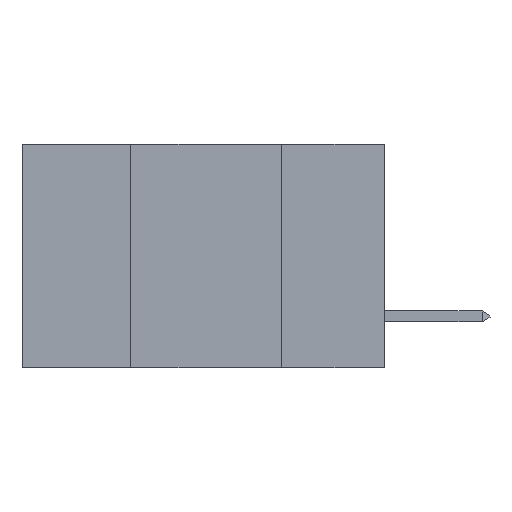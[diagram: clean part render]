
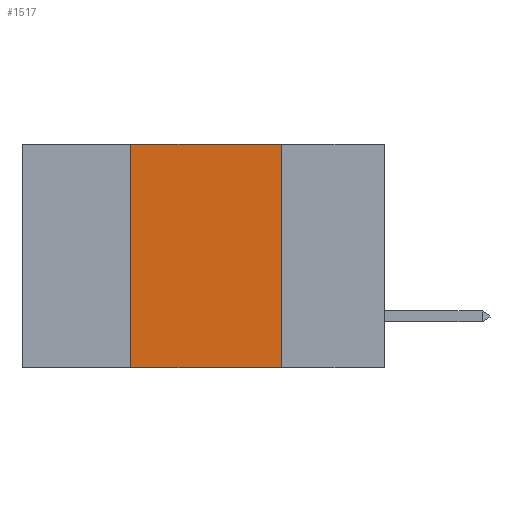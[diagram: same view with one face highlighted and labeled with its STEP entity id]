
A CAD part, left-side view. The second image highlights one B-rep face of the part: STEP entity #1517.
In plain terms, the highlighted planar face has unit normal (-1, 0, 0).
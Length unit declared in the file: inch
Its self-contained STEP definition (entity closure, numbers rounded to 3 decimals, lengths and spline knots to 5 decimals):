
#461 = CARTESIAN_POINT ( 'NONE',  ( 0., 0.6, 0. ) ) ;
#580 = EDGE_CURVE ( 'NONE', #10072, #6697, #18941, .T. ) ;
#1517 = ADVANCED_FACE ( 'NONE', ( #11629 ), #19166, .F. ) ;
#2607 = CARTESIAN_POINT ( 'NONE',  ( 0., 0.42, 0. ) ) ;
#3181 = VECTOR ( 'NONE', #10571, 39.37008 ) ;
#3670 = LINE ( 'NONE', #6433, #8417 ) ;
#4183 = EDGE_CURVE ( 'NONE', #6176, #10072, #11849, .T. ) ;
#5611 = DIRECTION ( 'NONE',  ( 0., -1., 0. ) ) ;
#6176 = VERTEX_POINT ( 'NONE', #2607 ) ;
#6433 = CARTESIAN_POINT ( 'NONE',  ( 0., 0.6, -0.37 ) ) ;
#6697 = VERTEX_POINT ( 'NONE', #12867 ) ;
#7623 = VECTOR ( 'NONE', #19845, 39.37008 ) ;
#8417 = VECTOR ( 'NONE', #20588, 39.37008 ) ;
#8633 = CARTESIAN_POINT ( 'NONE',  ( 0., 0.42, 0. ) ) ;
#8775 = ORIENTED_EDGE ( 'NONE', *, *, #20152, .F. ) ;
#9837 = ORIENTED_EDGE ( 'NONE', *, *, #13839, .T. ) ;
#10072 = VERTEX_POINT ( 'NONE', #19743 ) ;
#10571 = DIRECTION ( 'NONE',  ( 0., 0., -1. ) ) ;
#11629 = FACE_OUTER_BOUND ( 'NONE', #12415, .T. ) ;
#11849 = LINE ( 'NONE', #461, #19864 ) ;
#11900 = LINE ( 'NONE', #8633, #7623 ) ;
#12415 = EDGE_LOOP ( 'NONE', ( #15309, #13995, #8775, #9837 ) ) ;
#12867 = CARTESIAN_POINT ( 'NONE',  ( 0., 0.17, -0.37 ) ) ;
#13110 = AXIS2_PLACEMENT_3D ( 'NONE', #20757, #19586, #16432 ) ;
#13775 = VERTEX_POINT ( 'NONE', #18920 ) ;
#13839 = EDGE_CURVE ( 'NONE', #13775, #6697, #3670, .T. ) ;
#13995 = ORIENTED_EDGE ( 'NONE', *, *, #4183, .F. ) ;
#15309 = ORIENTED_EDGE ( 'NONE', *, *, #580, .F. ) ;
#16432 = DIRECTION ( 'NONE',  ( 0., 0., -1. ) ) ;
#18750 = CARTESIAN_POINT ( 'NONE',  ( 0., 0.17, 0. ) ) ;
#18920 = CARTESIAN_POINT ( 'NONE',  ( 0., 0.42, -0.37 ) ) ;
#18941 = LINE ( 'NONE', #18750, #3181 ) ;
#19166 = PLANE ( 'NONE',  #13110 ) ;
#19586 = DIRECTION ( 'NONE',  ( 1., 0., 0. ) ) ;
#19743 = CARTESIAN_POINT ( 'NONE',  ( 0., 0.17, 0. ) ) ;
#19845 = DIRECTION ( 'NONE',  ( 0., 0., 1. ) ) ;
#19864 = VECTOR ( 'NONE', #5611, 39.37008 ) ;
#20152 = EDGE_CURVE ( 'NONE', #13775, #6176, #11900, .T. ) ;
#20588 = DIRECTION ( 'NONE',  ( 0., -1., 0. ) ) ;
#20757 = CARTESIAN_POINT ( 'NONE',  ( 0., 0.6, 0. ) ) ;
